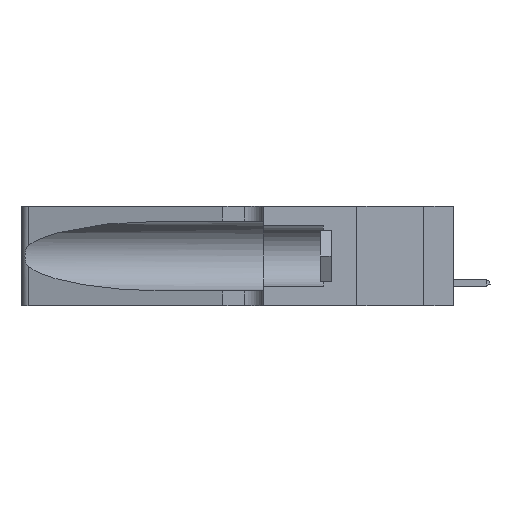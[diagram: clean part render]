
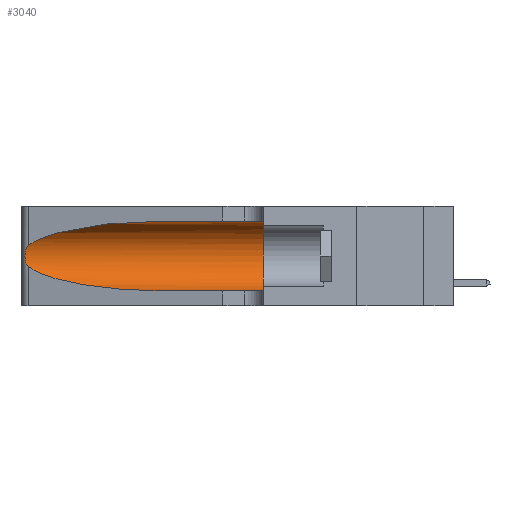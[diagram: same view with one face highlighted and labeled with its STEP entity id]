
A CAD part, left-side view. The second image highlights one B-rep face of the part: STEP entity #3040.
In plain terms, the highlighted cylindrical face has radius 3.308 mm (diameter 6.617 mm), a partial arc.
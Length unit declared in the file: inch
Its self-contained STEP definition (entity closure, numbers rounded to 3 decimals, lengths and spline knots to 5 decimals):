
#5 = CARTESIAN_POINT ( 'NONE',  ( 0.2373, 1.15595, 0.08982 ) ) ;
#212 =( BOUNDED_CURVE ( )  B_SPLINE_CURVE ( 3, ( #15634, #5, #4984, #18020 ),
 .UNSPECIFIED., .F., .F. ) 
 B_SPLINE_CURVE_WITH_KNOTS ( ( 4, 4 ),
 ( 3.44316, 4.71239 ),
 .UNSPECIFIED. ) 
 CURVE ( )  GEOMETRIC_REPRESENTATION_ITEM ( )  RATIONAL_B_SPLINE_CURVE ( ( 1., 0.87, 0.87, 1. ) ) 
 REPRESENTATION_ITEM ( '' )  );
#958 = ORIENTED_EDGE ( 'NONE', *, *, #2650, .T. ) ;
#2650 = EDGE_CURVE ( 'NONE', #31981, #15169, #212, .T. ) ;
#3040 = ADVANCED_FACE ( 'NONE', ( #33315 ), #3399, .F. ) ;
#3398 = CARTESIAN_POINT ( 'NONE',  ( 0.25487, 1.22718, 0.22369 ) ) ;
#3399 = CYLINDRICAL_SURFACE ( 'NONE', #19636, 0.13025 ) ;
#3997 = VECTOR ( 'NONE', #13978, 39.37008 ) ;
#4984 = CARTESIAN_POINT ( 'NONE',  ( 0.18966, 0.96281, 0.05475 ) ) ;
#5469 = ORIENTED_EDGE ( 'NONE', *, *, #8742, .T. ) ;
#6537 = VERTEX_POINT ( 'NONE', #18671 ) ;
#7728 = ORIENTED_EDGE ( 'NONE', *, *, #32672, .T. ) ;
#8720 = CARTESIAN_POINT ( 'NONE',  ( 0.25555, 1.22994, 0.2215 ) ) ;
#8742 = EDGE_CURVE ( 'NONE', #24208, #31981, #29743, .T. ) ;
#8940 = CARTESIAN_POINT ( 'NONE',  ( 0.25639, 1.23184, 0.21858 ) ) ;
#9103 = EDGE_CURVE ( 'NONE', #6537, #16216, #13226, .T. ) ;
#10653 = CARTESIAN_POINT ( 'NONE',  ( 0.2373, 1.15595, 0.28018 ) ) ;
#11357 = CARTESIAN_POINT ( 'NONE',  ( 0.1305, 1.61858, 0.31525 ) ) ;
#11386 = EDGE_CURVE ( 'NONE', #15169, #16216, #11412, .T. ) ;
#11412 = LINE ( 'NONE', #30655, #29423 ) ;
#11468 = ORIENTED_EDGE ( 'NONE', *, *, #17005, .F. ) ;
#12795 = DIRECTION ( 'NONE',  ( 0., 0., -1. ) ) ;
#13226 = CIRCLE ( 'NONE', #16265, 0.13025 ) ;
#13755 = CARTESIAN_POINT ( 'NONE',  ( 0.26017, 1.23833, 0.17102 ) ) ;
#13967 = CARTESIAN_POINT ( 'NONE',  ( 0.26075, 1.23896, 0.19203 ) ) ;
#13978 = DIRECTION ( 'NONE',  ( 0., -1., 0. ) ) ;
#15104 = DIRECTION ( 'NONE',  ( 0., 0., 1. ) ) ;
#15123 = DIRECTION ( 'NONE',  ( 0., -1., 0. ) ) ;
#15169 = VERTEX_POINT ( 'NONE', #31922 ) ;
#15634 = CARTESIAN_POINT ( 'NONE',  ( 0.25487, 1.22718, 0.14631 ) ) ;
#16216 = VERTEX_POINT ( 'NONE', #25541 ) ;
#16265 = AXIS2_PLACEMENT_3D ( 'NONE', #30795, #20198, #15104 ) ;
#16407 = CARTESIAN_POINT ( 'NONE',  ( 0.25856, 1.23593, 0.16098 ) ) ;
#17005 = EDGE_CURVE ( 'NONE', #27870, #6537, #24047, .T. ) ;
#18020 = CARTESIAN_POINT ( 'NONE',  ( 0.1305, 0.72297, 0.05475 ) ) ;
#18671 = CARTESIAN_POINT ( 'NONE',  ( 0.1305, 0.35, 0.31525 ) ) ;
#18998 = CARTESIAN_POINT ( 'NONE',  ( 0.25789, 1.23486, 0.15765 ) ) ;
#19115 = CARTESIAN_POINT ( 'NONE',  ( 0.26075, 1.23896, 0.178 ) ) ;
#19345 = CARTESIAN_POINT ( 'NONE',  ( 0.25854, 1.2359, 0.20912 ) ) ;
#19636 = AXIS2_PLACEMENT_3D ( 'NONE', #25955, #15123, #12795 ) ;
#19695 = EDGE_LOOP ( 'NONE', ( #7728, #5469, #958, #33319, #20788, #11468 ) ) ;
#20198 = DIRECTION ( 'NONE',  ( 0., 1., 0. ) ) ;
#20460 =( BOUNDED_CURVE ( )  B_SPLINE_CURVE ( 3, ( #31985, #23682, #10653, #26325 ),
 .UNSPECIFIED., .F., .T. ) 
 B_SPLINE_CURVE_WITH_KNOTS ( ( 4, 4 ),
 ( 1.5708, 2.84003 ),
 .UNSPECIFIED. ) 
 CURVE ( )  GEOMETRIC_REPRESENTATION_ITEM ( )  RATIONAL_B_SPLINE_CURVE ( ( 1., 0.87, 0.87, 1. ) ) 
 REPRESENTATION_ITEM ( '' )  );
#20688 = CARTESIAN_POINT ( 'NONE',  ( 0.25487, 1.22718, 0.22369 ) ) ;
#20788 = ORIENTED_EDGE ( 'NONE', *, *, #9103, .F. ) ;
#20886 = CARTESIAN_POINT ( 'NONE',  ( 0.1305, 0.72297, 0.31525 ) ) ;
#22040 = CARTESIAN_POINT ( 'NONE',  ( 0.26018, 1.23835, 0.19895 ) ) ;
#22399 = CARTESIAN_POINT ( 'NONE',  ( 0.25555, 1.22993, 0.14849 ) ) ;
#22629 = CARTESIAN_POINT ( 'NONE',  ( 0.25487, 1.22718, 0.14631 ) ) ;
#23682 = CARTESIAN_POINT ( 'NONE',  ( 0.18966, 0.96281, 0.31525 ) ) ;
#24047 = LINE ( 'NONE', #11357, #3997 ) ;
#24208 = VERTEX_POINT ( 'NONE', #3398 ) ;
#25541 = CARTESIAN_POINT ( 'NONE',  ( 0.1305, 0.35, 0.05475 ) ) ;
#25955 = CARTESIAN_POINT ( 'NONE',  ( 0.1305, 1.61858, 0.185 ) ) ;
#26030 = DIRECTION ( 'NONE',  ( 0., -1., 0. ) ) ;
#26140 = CARTESIAN_POINT ( 'NONE',  ( 0.25487, 1.22718, 0.14631 ) ) ;
#26325 = CARTESIAN_POINT ( 'NONE',  ( 0.25487, 1.22718, 0.22369 ) ) ;
#26907 = CARTESIAN_POINT ( 'NONE',  ( 0.25787, 1.23484, 0.2124 ) ) ;
#27870 = VERTEX_POINT ( 'NONE', #20886 ) ;
#29423 = VECTOR ( 'NONE', #26030, 39.37008 ) ;
#29743 = B_SPLINE_CURVE_WITH_KNOTS ( 'NONE', 3,
 ( #20688, #8720, #8940, #26907, #19345, #22040, #13967, #19115, #13755, #16407, #18998, #30133, #22399, #22629 ),
 .UNSPECIFIED., .F., .F.,
 ( 4, 2, 2, 2, 2, 2, 4 ),
 ( 0., 0.00027, 0.00053, 0.00107, 0.0016, 0.00187, 0.00214 ),
 .UNSPECIFIED. ) ;
#30133 = CARTESIAN_POINT ( 'NONE',  ( 0.25639, 1.23186, 0.15144 ) ) ;
#30655 = CARTESIAN_POINT ( 'NONE',  ( 0.1305, 1.61858, 0.05475 ) ) ;
#30795 = CARTESIAN_POINT ( 'NONE',  ( 0.1305, 0.35, 0.185 ) ) ;
#31922 = CARTESIAN_POINT ( 'NONE',  ( 0.1305, 0.72297, 0.05475 ) ) ;
#31981 = VERTEX_POINT ( 'NONE', #26140 ) ;
#31985 = CARTESIAN_POINT ( 'NONE',  ( 0.1305, 0.72297, 0.31525 ) ) ;
#32672 = EDGE_CURVE ( 'NONE', #27870, #24208, #20460, .T. ) ;
#33315 = FACE_OUTER_BOUND ( 'NONE', #19695, .T. ) ;
#33319 = ORIENTED_EDGE ( 'NONE', *, *, #11386, .T. ) ;
